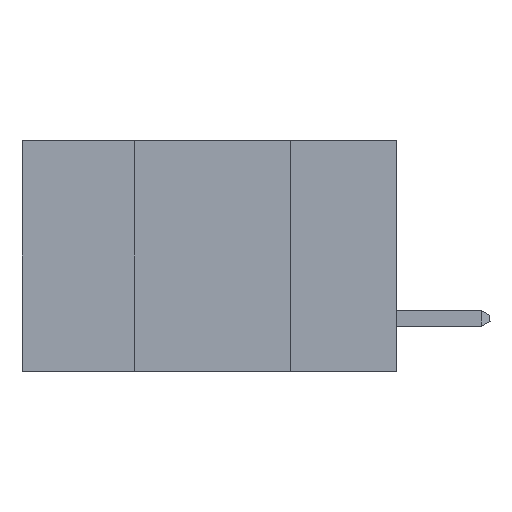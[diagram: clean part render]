
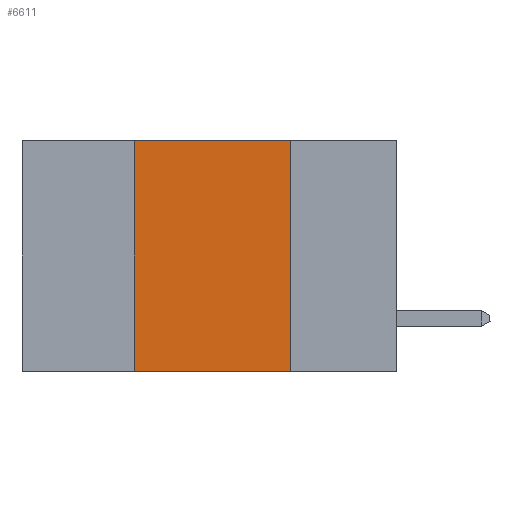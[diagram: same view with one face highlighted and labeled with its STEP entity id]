
A CAD part, left-side view. The second image highlights one B-rep face of the part: STEP entity #6611.
In plain terms, the highlighted planar face has unit normal (-1, 0, 0).
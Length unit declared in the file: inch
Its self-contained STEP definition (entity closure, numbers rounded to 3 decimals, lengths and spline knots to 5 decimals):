
#1267 = CARTESIAN_POINT ( 'NONE',  ( 0., 0.42, 0. ) ) ;
#1270 = CARTESIAN_POINT ( 'NONE',  ( 0., 0.6, 0. ) ) ;
#1794 = CARTESIAN_POINT ( 'NONE',  ( 0., 0.17, -0.37 ) ) ;
#1831 = AXIS2_PLACEMENT_3D ( 'NONE', #10052, #9028, #7976 ) ;
#2353 = DIRECTION ( 'NONE',  ( 0., 0., -1. ) ) ;
#2473 = VECTOR ( 'NONE', #2353, 39.37008 ) ;
#2515 = CARTESIAN_POINT ( 'NONE',  ( 0., 0.17, 0. ) ) ;
#3216 = CARTESIAN_POINT ( 'NONE',  ( 0., 0.17, 0. ) ) ;
#3296 = DIRECTION ( 'NONE',  ( 0., -1., 0. ) ) ;
#3457 = ORIENTED_EDGE ( 'NONE', *, *, #4782, .T. ) ;
#4022 = LINE ( 'NONE', #1270, #11949 ) ;
#4100 = LINE ( 'NONE', #7153, #12667 ) ;
#4238 = DIRECTION ( 'NONE',  ( 0., 0., 1. ) ) ;
#4782 = EDGE_CURVE ( 'NONE', #6778, #10102, #4100, .T. ) ;
#5065 = DIRECTION ( 'NONE',  ( 0., -1., 0. ) ) ;
#5167 = ORIENTED_EDGE ( 'NONE', *, *, #8304, .F. ) ;
#5490 = CARTESIAN_POINT ( 'NONE',  ( 0., 0.42, 0. ) ) ;
#6611 = ADVANCED_FACE ( 'NONE', ( #9334 ), #6987, .F. ) ;
#6778 = VERTEX_POINT ( 'NONE', #12488 ) ;
#6783 = EDGE_CURVE ( 'NONE', #10926, #10102, #10429, .T. ) ;
#6987 = PLANE ( 'NONE',  #1831 ) ;
#7153 = CARTESIAN_POINT ( 'NONE',  ( 0., 0.6, -0.37 ) ) ;
#7410 = EDGE_LOOP ( 'NONE', ( #7631, #10625, #5167, #3457 ) ) ;
#7481 = VERTEX_POINT ( 'NONE', #1267 ) ;
#7631 = ORIENTED_EDGE ( 'NONE', *, *, #6783, .F. ) ;
#7976 = DIRECTION ( 'NONE',  ( 0., 0., -1. ) ) ;
#8304 = EDGE_CURVE ( 'NONE', #6778, #7481, #10079, .T. ) ;
#9028 = DIRECTION ( 'NONE',  ( 1., 0., 0. ) ) ;
#9334 = FACE_OUTER_BOUND ( 'NONE', #7410, .T. ) ;
#9807 = EDGE_CURVE ( 'NONE', #7481, #10926, #4022, .T. ) ;
#10052 = CARTESIAN_POINT ( 'NONE',  ( 0., 0.6, 0. ) ) ;
#10079 = LINE ( 'NONE', #5490, #12401 ) ;
#10102 = VERTEX_POINT ( 'NONE', #1794 ) ;
#10429 = LINE ( 'NONE', #3216, #2473 ) ;
#10625 = ORIENTED_EDGE ( 'NONE', *, *, #9807, .F. ) ;
#10926 = VERTEX_POINT ( 'NONE', #2515 ) ;
#11949 = VECTOR ( 'NONE', #3296, 39.37008 ) ;
#12401 = VECTOR ( 'NONE', #4238, 39.37008 ) ;
#12488 = CARTESIAN_POINT ( 'NONE',  ( 0., 0.42, -0.37 ) ) ;
#12667 = VECTOR ( 'NONE', #5065, 39.37008 ) ;
